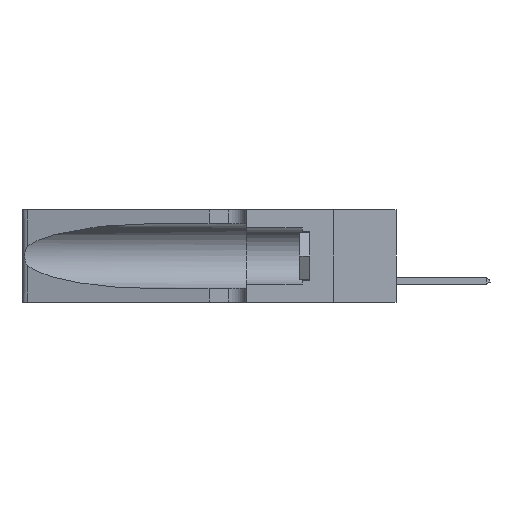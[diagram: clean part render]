
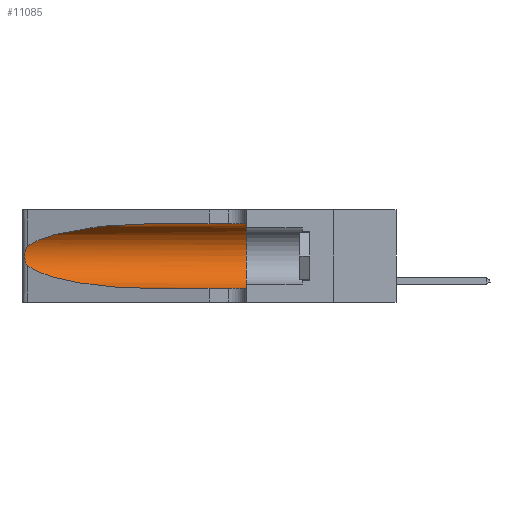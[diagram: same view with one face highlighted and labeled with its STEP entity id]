
A CAD part, left-side view. The second image highlights one B-rep face of the part: STEP entity #11085.
In plain terms, the highlighted cylindrical face has radius 3.308 mm (diameter 6.617 mm), a partial arc.
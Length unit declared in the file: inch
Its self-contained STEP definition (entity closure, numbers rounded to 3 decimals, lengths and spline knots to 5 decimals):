
#74 = CARTESIAN_POINT ( 'NONE',  ( 0.25639, 1.23184, 0.21858 ) ) ;
#814 = EDGE_CURVE ( 'NONE', #18646, #20451, #2979, .T. ) ;
#878 = CARTESIAN_POINT ( 'NONE',  ( 0.26075, 1.23896, 0.178 ) ) ;
#922 = CARTESIAN_POINT ( 'NONE',  ( 0.25487, 1.22718, 0.22369 ) ) ;
#1106 = CARTESIAN_POINT ( 'NONE',  ( 0.18966, 0.96281, 0.05475 ) ) ;
#1117 = EDGE_CURVE ( 'NONE', #20451, #9704, #17320, .T. ) ;
#2528 = CARTESIAN_POINT ( 'NONE',  ( 0.18966, 0.96281, 0.31525 ) ) ;
#2676 = CARTESIAN_POINT ( 'NONE',  ( 0.1305, 0.35, 0.05475 ) ) ;
#2979 =( BOUNDED_CURVE ( )  B_SPLINE_CURVE ( 3, ( #11166, #2528, #5864, #922 ),
 .UNSPECIFIED., .F., .F. ) 
 B_SPLINE_CURVE_WITH_KNOTS ( ( 4, 4 ),
 ( 1.5708, 2.84003 ),
 .UNSPECIFIED. ) 
 CURVE ( )  GEOMETRIC_REPRESENTATION_ITEM ( )  RATIONAL_B_SPLINE_CURVE ( ( 1., 0.87, 0.87, 1. ) ) 
 REPRESENTATION_ITEM ( '' )  );
#3155 = CARTESIAN_POINT ( 'NONE',  ( 0.26018, 1.23835, 0.19895 ) ) ;
#4134 = CARTESIAN_POINT ( 'NONE',  ( 0.25487, 1.22718, 0.14631 ) ) ;
#4235 = ORIENTED_EDGE ( 'NONE', *, *, #11277, .F. ) ;
#4659 = CARTESIAN_POINT ( 'NONE',  ( 0.25487, 1.22718, 0.14631 ) ) ;
#4828 = CARTESIAN_POINT ( 'NONE',  ( 0.1305, 1.61858, 0.31525 ) ) ;
#5106 = CARTESIAN_POINT ( 'NONE',  ( 0.25787, 1.23484, 0.2124 ) ) ;
#5347 = DIRECTION ( 'NONE',  ( 0., 0., 1. ) ) ;
#5864 = CARTESIAN_POINT ( 'NONE',  ( 0.2373, 1.15595, 0.28018 ) ) ;
#5880 = CARTESIAN_POINT ( 'NONE',  ( 0.25856, 1.23593, 0.16098 ) ) ;
#5934 = AXIS2_PLACEMENT_3D ( 'NONE', #13650, #6995, #5347 ) ;
#6291 = VERTEX_POINT ( 'NONE', #2676 ) ;
#6449 = FACE_OUTER_BOUND ( 'NONE', #11478, .T. ) ;
#6495 = CARTESIAN_POINT ( 'NONE',  ( 0.26075, 1.23896, 0.19203 ) ) ;
#6742 = CARTESIAN_POINT ( 'NONE',  ( 0.1305, 1.61858, 0.05475 ) ) ;
#6995 = DIRECTION ( 'NONE',  ( 0., 1., 0. ) ) ;
#7122 = EDGE_CURVE ( 'NONE', #18646, #12710, #19008, .T. ) ;
#7920 = ORIENTED_EDGE ( 'NONE', *, *, #21419, .T. ) ;
#8163 = DIRECTION ( 'NONE',  ( 0., -1., 0. ) ) ;
#8234 = CYLINDRICAL_SURFACE ( 'NONE', #20300, 0.13025 ) ;
#8661 = VECTOR ( 'NONE', #8163, 39.37008 ) ;
#9100 = CARTESIAN_POINT ( 'NONE',  ( 0.25487, 1.22718, 0.14631 ) ) ;
#9304 = ORIENTED_EDGE ( 'NONE', *, *, #1117, .T. ) ;
#9522 = CARTESIAN_POINT ( 'NONE',  ( 0.2373, 1.15595, 0.08982 ) ) ;
#9525 = ORIENTED_EDGE ( 'NONE', *, *, #7122, .F. ) ;
#9704 = VERTEX_POINT ( 'NONE', #4134 ) ;
#9994 = CARTESIAN_POINT ( 'NONE',  ( 0.25487, 1.22718, 0.22369 ) ) ;
#10315 = ORIENTED_EDGE ( 'NONE', *, *, #814, .T. ) ;
#10839 = CARTESIAN_POINT ( 'NONE',  ( 0.1305, 1.61858, 0.185 ) ) ;
#11085 = ADVANCED_FACE ( 'NONE', ( #6449 ), #8234, .F. ) ;
#11166 = CARTESIAN_POINT ( 'NONE',  ( 0.1305, 0.72297, 0.31525 ) ) ;
#11277 = EDGE_CURVE ( 'NONE', #12710, #6291, #13664, .T. ) ;
#11478 = EDGE_LOOP ( 'NONE', ( #10315, #9304, #7920, #17564, #4235, #9525 ) ) ;
#12276 = VERTEX_POINT ( 'NONE', #12328 ) ;
#12328 = CARTESIAN_POINT ( 'NONE',  ( 0.1305, 0.72297, 0.05475 ) ) ;
#12375 = DIRECTION ( 'NONE',  ( 0., -1., 0. ) ) ;
#12434 = CARTESIAN_POINT ( 'NONE',  ( 0.26017, 1.23833, 0.17102 ) ) ;
#12710 = VERTEX_POINT ( 'NONE', #13460 ) ;
#12769 = CARTESIAN_POINT ( 'NONE',  ( 0.25487, 1.22718, 0.22369 ) ) ;
#13460 = CARTESIAN_POINT ( 'NONE',  ( 0.1305, 0.35, 0.31525 ) ) ;
#13650 = CARTESIAN_POINT ( 'NONE',  ( 0.1305, 0.35, 0.185 ) ) ;
#13664 = CIRCLE ( 'NONE', #5934, 0.13025 ) ;
#14400 = CARTESIAN_POINT ( 'NONE',  ( 0.1305, 0.72297, 0.05475 ) ) ;
#15518 = EDGE_CURVE ( 'NONE', #12276, #6291, #20564, .T. ) ;
#15777 = DIRECTION ( 'NONE',  ( 0., 0., -1. ) ) ;
#16091 = CARTESIAN_POINT ( 'NONE',  ( 0.25555, 1.22994, 0.2215 ) ) ;
#17064 = CARTESIAN_POINT ( 'NONE',  ( 0.1305, 0.72297, 0.31525 ) ) ;
#17320 = B_SPLINE_CURVE_WITH_KNOTS ( 'NONE', 3,
 ( #12769, #16091, #74, #5106, #18099, #3155, #6495, #878, #12434, #5880, #17431, #17371, #19009, #9100 ),
 .UNSPECIFIED., .F., .F.,
 ( 4, 2, 2, 2, 2, 2, 4 ),
 ( 0., 0.00027, 0.00053, 0.00107, 0.0016, 0.00187, 0.00214 ),
 .UNSPECIFIED. ) ;
#17371 = CARTESIAN_POINT ( 'NONE',  ( 0.25639, 1.23186, 0.15144 ) ) ;
#17431 = CARTESIAN_POINT ( 'NONE',  ( 0.25789, 1.23486, 0.15765 ) ) ;
#17564 = ORIENTED_EDGE ( 'NONE', *, *, #15518, .T. ) ;
#18099 = CARTESIAN_POINT ( 'NONE',  ( 0.25854, 1.2359, 0.20912 ) ) ;
#18646 = VERTEX_POINT ( 'NONE', #17064 ) ;
#19008 = LINE ( 'NONE', #4828, #8661 ) ;
#19009 = CARTESIAN_POINT ( 'NONE',  ( 0.25555, 1.22993, 0.14849 ) ) ;
#19932 = DIRECTION ( 'NONE',  ( 0., -1., 0. ) ) ;
#20203 =( BOUNDED_CURVE ( )  B_SPLINE_CURVE ( 3, ( #4659, #9522, #1106, #14400 ),
 .UNSPECIFIED., .F., .F. ) 
 B_SPLINE_CURVE_WITH_KNOTS ( ( 4, 4 ),
 ( 3.44316, 4.71239 ),
 .UNSPECIFIED. ) 
 CURVE ( )  GEOMETRIC_REPRESENTATION_ITEM ( )  RATIONAL_B_SPLINE_CURVE ( ( 1., 0.87, 0.87, 1. ) ) 
 REPRESENTATION_ITEM ( '' )  );
#20296 = VECTOR ( 'NONE', #19932, 39.37008 ) ;
#20300 = AXIS2_PLACEMENT_3D ( 'NONE', #10839, #12375, #15777 ) ;
#20451 = VERTEX_POINT ( 'NONE', #9994 ) ;
#20564 = LINE ( 'NONE', #6742, #20296 ) ;
#21419 = EDGE_CURVE ( 'NONE', #9704, #12276, #20203, .T. ) ;
